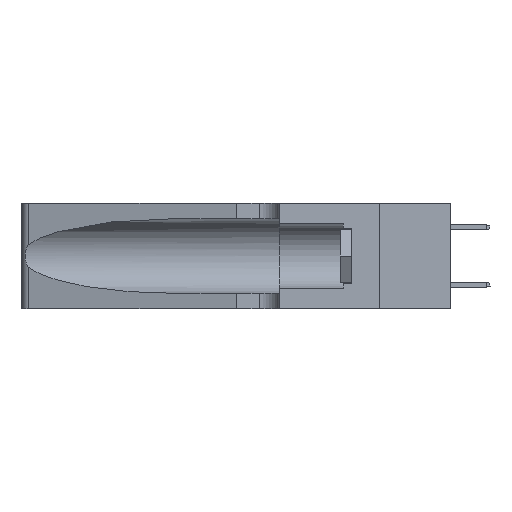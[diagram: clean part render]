
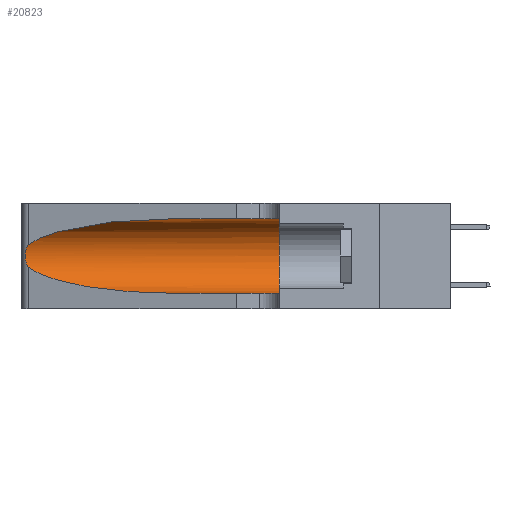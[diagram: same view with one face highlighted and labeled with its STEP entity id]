
A CAD part, left-side view. The second image highlights one B-rep face of the part: STEP entity #20823.
In plain terms, the highlighted cylindrical face has radius 3.308 mm (diameter 6.617 mm), a partial arc.
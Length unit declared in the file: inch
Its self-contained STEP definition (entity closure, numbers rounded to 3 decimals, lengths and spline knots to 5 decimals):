
#472 = CARTESIAN_POINT ( 'NONE',  ( 0.1305, 0.72297, 0.31525 ) ) ;
#1915 = CARTESIAN_POINT ( 'NONE',  ( 0.25487, 1.22718, 0.14631 ) ) ;
#1977 = ORIENTED_EDGE ( 'NONE', *, *, #13668, .T. ) ;
#2073 = DIRECTION ( 'NONE',  ( 0., 1., 0. ) ) ;
#2167 = LINE ( 'NONE', #11455, #20172 ) ;
#2395 = EDGE_CURVE ( 'NONE', #21864, #7008, #2167, .T. ) ;
#3392 = EDGE_LOOP ( 'NONE', ( #13344, #1977, #21447, #16750, #17206, #26852 ) ) ;
#3940 = CARTESIAN_POINT ( 'NONE',  ( 0.25789, 1.23486, 0.15765 ) ) ;
#4304 = VERTEX_POINT ( 'NONE', #14445 ) ;
#4371 = CARTESIAN_POINT ( 'NONE',  ( 0.1305, 0.35, 0.185 ) ) ;
#5317 = LINE ( 'NONE', #14598, #28423 ) ;
#5343 = CYLINDRICAL_SURFACE ( 'NONE', #29151, 0.13025 ) ;
#5625 = EDGE_CURVE ( 'NONE', #14821, #4304, #28416, .T. ) ;
#6082 = CARTESIAN_POINT ( 'NONE',  ( 0.25787, 1.23484, 0.2124 ) ) ;
#7008 = VERTEX_POINT ( 'NONE', #13202 ) ;
#7057 = CARTESIAN_POINT ( 'NONE',  ( 0.18966, 0.96281, 0.31525 ) ) ;
#8311 = CIRCLE ( 'NONE', #21905, 0.13025 ) ;
#9443 = DIRECTION ( 'NONE',  ( 0., -1., 0. ) ) ;
#9587 = DIRECTION ( 'NONE',  ( 0., 0., -1. ) ) ;
#10465 = EDGE_CURVE ( 'NONE', #14821, #25539, #5317, .T. ) ;
#10485 = CARTESIAN_POINT ( 'NONE',  ( 0.25487, 1.22718, 0.22369 ) ) ;
#11190 = CARTESIAN_POINT ( 'NONE',  ( 0.18966, 0.96281, 0.05475 ) ) ;
#11359 = DIRECTION ( 'NONE',  ( 0., 0., 1. ) ) ;
#11455 = CARTESIAN_POINT ( 'NONE',  ( 0.1305, 1.61858, 0.05475 ) ) ;
#12640 = CARTESIAN_POINT ( 'NONE',  ( 0.25854, 1.2359, 0.20912 ) ) ;
#13202 = CARTESIAN_POINT ( 'NONE',  ( 0.1305, 0.35, 0.05475 ) ) ;
#13344 = ORIENTED_EDGE ( 'NONE', *, *, #5625, .T. ) ;
#13668 = EDGE_CURVE ( 'NONE', #4304, #20113, #20287, .T. ) ;
#14445 = CARTESIAN_POINT ( 'NONE',  ( 0.25487, 1.22718, 0.22369 ) ) ;
#14459 = FACE_OUTER_BOUND ( 'NONE', #3392, .T. ) ;
#14598 = CARTESIAN_POINT ( 'NONE',  ( 0.1305, 1.61858, 0.31525 ) ) ;
#14821 = VERTEX_POINT ( 'NONE', #472 ) ;
#15213 = CARTESIAN_POINT ( 'NONE',  ( 0.25639, 1.23184, 0.21858 ) ) ;
#15348 = CARTESIAN_POINT ( 'NONE',  ( 0.26075, 1.23896, 0.178 ) ) ;
#15503 = CARTESIAN_POINT ( 'NONE',  ( 0.26075, 1.23896, 0.19203 ) ) ;
#16185 = CARTESIAN_POINT ( 'NONE',  ( 0.1305, 0.72297, 0.31525 ) ) ;
#16221 = CARTESIAN_POINT ( 'NONE',  ( 0.1305, 0.72297, 0.05475 ) ) ;
#16750 = ORIENTED_EDGE ( 'NONE', *, *, #2395, .T. ) ;
#17206 = ORIENTED_EDGE ( 'NONE', *, *, #21680, .F. ) ;
#17476 = CARTESIAN_POINT ( 'NONE',  ( 0.25555, 1.22994, 0.2215 ) ) ;
#19457 = CARTESIAN_POINT ( 'NONE',  ( 0.25555, 1.22993, 0.14849 ) ) ;
#19791 = EDGE_CURVE ( 'NONE', #20113, #21864, #26271, .T. ) ;
#20034 = CARTESIAN_POINT ( 'NONE',  ( 0.25639, 1.23186, 0.15144 ) ) ;
#20113 = VERTEX_POINT ( 'NONE', #20411 ) ;
#20172 = VECTOR ( 'NONE', #26922, 39.37008 ) ;
#20287 = B_SPLINE_CURVE_WITH_KNOTS ( 'NONE', 3,
 ( #10485, #17476, #15213, #6082, #12640, #21880, #15503, #15348, #28874, #26434, #3940, #20034, #19457, #24583 ),
 .UNSPECIFIED., .F., .F.,
 ( 4, 2, 2, 2, 2, 2, 4 ),
 ( 0., 0.00027, 0.00053, 0.00107, 0.0016, 0.00187, 0.00214 ),
 .UNSPECIFIED. ) ;
#20411 = CARTESIAN_POINT ( 'NONE',  ( 0.25487, 1.22718, 0.14631 ) ) ;
#20823 = ADVANCED_FACE ( 'NONE', ( #14459 ), #5343, .F. ) ;
#21447 = ORIENTED_EDGE ( 'NONE', *, *, #19791, .T. ) ;
#21680 = EDGE_CURVE ( 'NONE', #25539, #7008, #8311, .T. ) ;
#21864 = VERTEX_POINT ( 'NONE', #24190 ) ;
#21880 = CARTESIAN_POINT ( 'NONE',  ( 0.26018, 1.23835, 0.19895 ) ) ;
#21905 = AXIS2_PLACEMENT_3D ( 'NONE', #4371, #2073, #11359 ) ;
#23261 = CARTESIAN_POINT ( 'NONE',  ( 0.1305, 1.61858, 0.185 ) ) ;
#23994 = CARTESIAN_POINT ( 'NONE',  ( 0.2373, 1.15595, 0.28018 ) ) ;
#24190 = CARTESIAN_POINT ( 'NONE',  ( 0.1305, 0.72297, 0.05475 ) ) ;
#24583 = CARTESIAN_POINT ( 'NONE',  ( 0.25487, 1.22718, 0.14631 ) ) ;
#24988 = CARTESIAN_POINT ( 'NONE',  ( 0.1305, 0.35, 0.31525 ) ) ;
#25539 = VERTEX_POINT ( 'NONE', #24988 ) ;
#25550 = CARTESIAN_POINT ( 'NONE',  ( 0.25487, 1.22718, 0.22369 ) ) ;
#26258 = DIRECTION ( 'NONE',  ( 0., -1., 0. ) ) ;
#26271 =( BOUNDED_CURVE ( )  B_SPLINE_CURVE ( 3, ( #1915, #27434, #11190, #16221 ),
 .UNSPECIFIED., .F., .T. ) 
 B_SPLINE_CURVE_WITH_KNOTS ( ( 4, 4 ),
 ( 3.44316, 4.71239 ),
 .UNSPECIFIED. ) 
 CURVE ( )  GEOMETRIC_REPRESENTATION_ITEM ( )  RATIONAL_B_SPLINE_CURVE ( ( 1., 0.87, 0.87, 1. ) ) 
 REPRESENTATION_ITEM ( '' )  );
#26434 = CARTESIAN_POINT ( 'NONE',  ( 0.25856, 1.23593, 0.16098 ) ) ;
#26852 = ORIENTED_EDGE ( 'NONE', *, *, #10465, .F. ) ;
#26922 = DIRECTION ( 'NONE',  ( 0., -1., 0. ) ) ;
#27434 = CARTESIAN_POINT ( 'NONE',  ( 0.2373, 1.15595, 0.08982 ) ) ;
#28416 =( BOUNDED_CURVE ( )  B_SPLINE_CURVE ( 3, ( #16185, #7057, #23994, #25550 ),
 .UNSPECIFIED., .F., .T. ) 
 B_SPLINE_CURVE_WITH_KNOTS ( ( 4, 4 ),
 ( 1.5708, 2.84003 ),
 .UNSPECIFIED. ) 
 CURVE ( )  GEOMETRIC_REPRESENTATION_ITEM ( )  RATIONAL_B_SPLINE_CURVE ( ( 1., 0.87, 0.87, 1. ) ) 
 REPRESENTATION_ITEM ( '' )  );
#28423 = VECTOR ( 'NONE', #26258, 39.37008 ) ;
#28874 = CARTESIAN_POINT ( 'NONE',  ( 0.26017, 1.23833, 0.17102 ) ) ;
#29151 = AXIS2_PLACEMENT_3D ( 'NONE', #23261, #9443, #9587 ) ;
